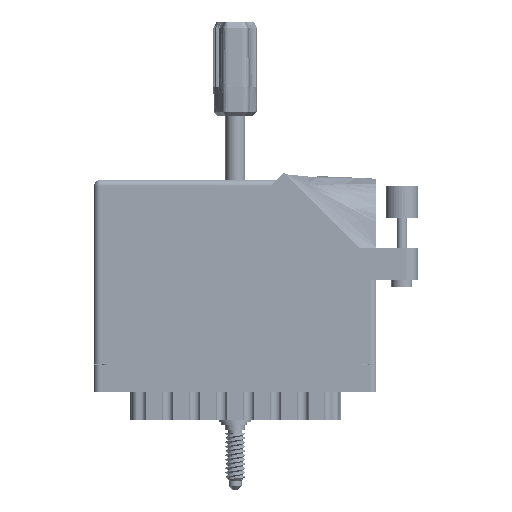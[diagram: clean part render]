
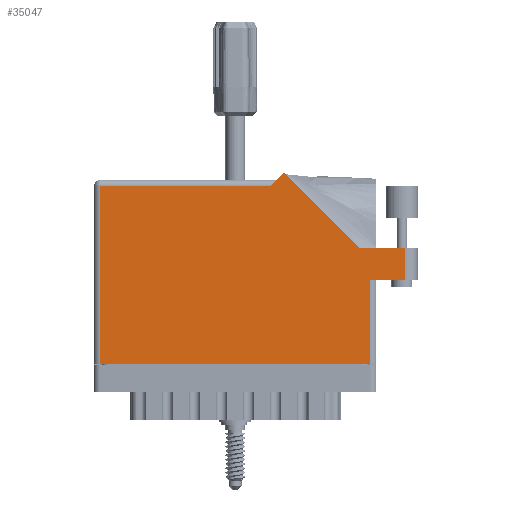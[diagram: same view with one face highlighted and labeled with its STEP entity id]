
A CAD part, front view. The second image highlights one B-rep face of the part: STEP entity #35047.
In plain terms, the highlighted face is planar.
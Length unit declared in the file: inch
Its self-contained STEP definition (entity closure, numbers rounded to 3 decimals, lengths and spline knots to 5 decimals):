
#225 = VECTOR ( 'NONE', #67161, 39.37008 ) ;
#797 = VERTEX_POINT ( 'NONE', #50457 ) ;
#2120 = EDGE_CURVE ( 'NONE', #10603, #41733, #64143, .T. ) ;
#2738 = EDGE_CURVE ( 'NONE', #14181, #25505, #44525, .T. ) ;
#2800 = VECTOR ( 'NONE', #26655, 39.37008 ) ;
#4983 = LINE ( 'NONE', #64339, #20087 ) ;
#7471 = LINE ( 'NONE', #71633, #37659 ) ;
#8775 = VECTOR ( 'NONE', #19944, 39.37008 ) ;
#9683 = ORIENTED_EDGE ( 'NONE', *, *, #55388, .T. ) ;
#10603 = VERTEX_POINT ( 'NONE', #52339 ) ;
#11590 = CARTESIAN_POINT ( 'NONE',  ( 0., 1.713, 0. ) ) ;
#13403 = ORIENTED_EDGE ( 'NONE', *, *, #2738, .T. ) ;
#14181 = VERTEX_POINT ( 'NONE', #68147 ) ;
#16095 = ORIENTED_EDGE ( 'NONE', *, *, #64924, .T. ) ;
#16785 = VERTEX_POINT ( 'NONE', #21003 ) ;
#17040 = CARTESIAN_POINT ( 'NONE',  ( 2.993, 1.122, 0. ) ) ;
#17406 = CARTESIAN_POINT ( 'NONE',  ( 2.656, 0.815, 0. ) ) ;
#18061 = PLANE ( 'NONE',  #40593 ) ;
#18191 = CARTESIAN_POINT ( 'NONE',  ( 1.758, 1.775, 0. ) ) ;
#18304 = DIRECTION ( 'NONE',  ( 0., 1., 0. ) ) ;
#19781 = CARTESIAN_POINT ( 'NONE',  ( 2.993, 1.122, 0. ) ) ;
#19944 = DIRECTION ( 'NONE',  ( -0.707, 0.707, 0. ) ) ;
#20087 = VECTOR ( 'NONE', #86005, 39.37008 ) ;
#21003 = CARTESIAN_POINT ( 'NONE',  ( 2.993, 0.815, 0. ) ) ;
#25251 = DIRECTION ( 'NONE',  ( -1., 0., 0. ) ) ;
#25505 = VERTEX_POINT ( 'NONE', #58789 ) ;
#25835 = DIRECTION ( 'NONE',  ( 1., 0., 0. ) ) ;
#26655 = DIRECTION ( 'NONE',  ( 0., 1., 0. ) ) ;
#27548 = EDGE_CURVE ( 'NONE', #25505, #68719, #87051, .T. ) ;
#30390 = EDGE_CURVE ( 'NONE', #62648, #58856, #61906, .T. ) ;
#33116 = CARTESIAN_POINT ( 'NONE',  ( 2.55242, 1.122, 0. ) ) ;
#33994 = CARTESIAN_POINT ( 'NONE',  ( 2.718, 0.815, 0. ) ) ;
#35047 = ADVANCED_FACE ( 'NONE', ( #54065 ), #18061, .F. ) ;
#35824 = VECTOR ( 'NONE', #67723, 39.37008 ) ;
#37119 = LINE ( 'NONE', #33994, #42511 ) ;
#37659 = VECTOR ( 'NONE', #85153, 39.37008 ) ;
#37951 = DIRECTION ( 'NONE',  ( 0., 0., -1. ) ) ;
#38115 = EDGE_CURVE ( 'NONE', #68719, #797, #4983, .T. ) ;
#40593 = AXIS2_PLACEMENT_3D ( 'NONE', #86909, #37951, #25251 ) ;
#41600 = VECTOR ( 'NONE', #73828, 39.37008 ) ;
#41610 = CARTESIAN_POINT ( 'NONE',  ( 2.55242, 1.122, 0. ) ) ;
#41733 = VERTEX_POINT ( 'NONE', #55196 ) ;
#42511 = VECTOR ( 'NONE', #25835, 39.37008 ) ;
#44525 = LINE ( 'NONE', #18191, #225 ) ;
#44622 = ORIENTED_EDGE ( 'NONE', *, *, #27548, .T. ) ;
#47455 = EDGE_LOOP ( 'NONE', ( #75700, #64067, #48175, #9683, #13403, #44622, #73800, #16095, #51998 ) ) ;
#48175 = ORIENTED_EDGE ( 'NONE', *, *, #30390, .T. ) ;
#50457 = CARTESIAN_POINT ( 'NONE',  ( 0.062, 0., 0. ) ) ;
#51080 = EDGE_CURVE ( 'NONE', #41733, #16785, #37119, .T. ) ;
#51998 = ORIENTED_EDGE ( 'NONE', *, *, #2120, .T. ) ;
#52339 = CARTESIAN_POINT ( 'NONE',  ( 2.656, 0., 0. ) ) ;
#54065 = FACE_OUTER_BOUND ( 'NONE', #47455, .T. ) ;
#54219 = LINE ( 'NONE', #41610, #8775 ) ;
#55196 = CARTESIAN_POINT ( 'NONE',  ( 2.656, 0.815, 0. ) ) ;
#55388 = EDGE_CURVE ( 'NONE', #58856, #14181, #54219, .T. ) ;
#58789 = CARTESIAN_POINT ( 'NONE',  ( 1.696, 1.713, 0. ) ) ;
#58856 = VERTEX_POINT ( 'NONE', #33116 ) ;
#61906 = LINE ( 'NONE', #82161, #35824 ) ;
#62291 = LINE ( 'NONE', #19781, #2800 ) ;
#62648 = VERTEX_POINT ( 'NONE', #17040 ) ;
#64067 = ORIENTED_EDGE ( 'NONE', *, *, #79377, .T. ) ;
#64143 = LINE ( 'NONE', #17406, #69479 ) ;
#64339 = CARTESIAN_POINT ( 'NONE',  ( 0.062, 0., 0. ) ) ;
#64924 = EDGE_CURVE ( 'NONE', #797, #10603, #7471, .T. ) ;
#67161 = DIRECTION ( 'NONE',  ( -0.707, -0.707, 0. ) ) ;
#67723 = DIRECTION ( 'NONE',  ( -1., 0., 0. ) ) ;
#68147 = CARTESIAN_POINT ( 'NONE',  ( 1.82871, 1.84571, 0. ) ) ;
#68719 = VERTEX_POINT ( 'NONE', #69919 ) ;
#69479 = VECTOR ( 'NONE', #18304, 39.37008 ) ;
#69919 = CARTESIAN_POINT ( 'NONE',  ( 0.062, 1.713, 0. ) ) ;
#71633 = CARTESIAN_POINT ( 'NONE',  ( 0., 0., 0. ) ) ;
#73800 = ORIENTED_EDGE ( 'NONE', *, *, #38115, .T. ) ;
#73828 = DIRECTION ( 'NONE',  ( -1., 0., 0. ) ) ;
#75700 = ORIENTED_EDGE ( 'NONE', *, *, #51080, .T. ) ;
#79377 = EDGE_CURVE ( 'NONE', #16785, #62648, #62291, .T. ) ;
#82161 = CARTESIAN_POINT ( 'NONE',  ( 3.118, 1.122, 0. ) ) ;
#85153 = DIRECTION ( 'NONE',  ( 1., 0., 0. ) ) ;
#86005 = DIRECTION ( 'NONE',  ( 0., -1., 0. ) ) ;
#86909 = CARTESIAN_POINT ( 'NONE',  ( 0., 1.775, 0. ) ) ;
#87051 = LINE ( 'NONE', #11590, #41600 ) ;
